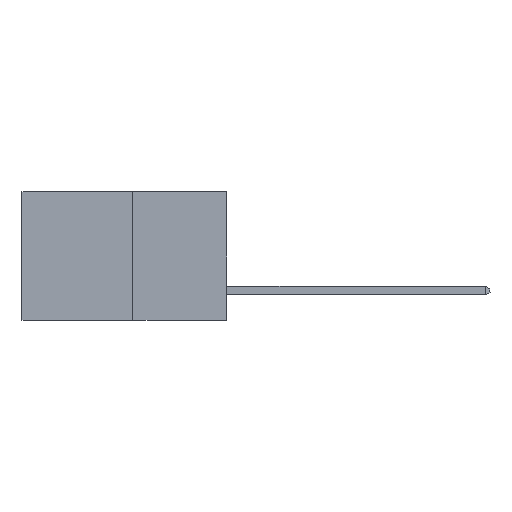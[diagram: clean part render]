
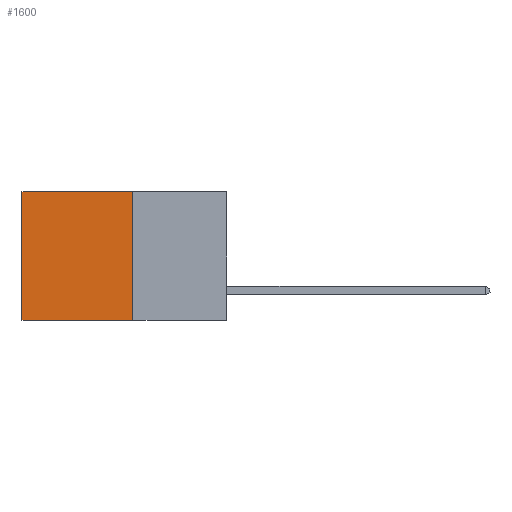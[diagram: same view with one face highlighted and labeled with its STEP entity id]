
A CAD part, left-side view. The second image highlights one B-rep face of the part: STEP entity #1600.
In plain terms, the highlighted planar face has unit normal (-1, 0, 0).
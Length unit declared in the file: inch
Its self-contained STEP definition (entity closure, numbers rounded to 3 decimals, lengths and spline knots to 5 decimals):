
#81 = EDGE_CURVE ( 'NONE', #3476, #1155, #4090, .T. ) ;
#1049 = ORIENTED_EDGE ( 'NONE', *, *, #2404, .T. ) ;
#1155 = VERTEX_POINT ( 'NONE', #3447 ) ;
#1250 = VECTOR ( 'NONE', #4417, 39.37008 ) ;
#1600 = ADVANCED_FACE ( 'NONE', ( #4902 ), #5461, .F. ) ;
#1651 = ORIENTED_EDGE ( 'NONE', *, *, #4720, .T. ) ;
#1663 = ORIENTED_EDGE ( 'NONE', *, *, #81, .F. ) ;
#1811 = VECTOR ( 'NONE', #3753, 39.37008 ) ;
#1872 = ORIENTED_EDGE ( 'NONE', *, *, #5780, .F. ) ;
#2404 = EDGE_CURVE ( 'NONE', #3476, #9478, #9103, .T. ) ;
#2645 = VECTOR ( 'NONE', #2736, 39.37008 ) ;
#2736 = DIRECTION ( 'NONE',  ( 0., 1., 0. ) ) ;
#3257 = VECTOR ( 'NONE', #9113, 39.37008 ) ;
#3447 = CARTESIAN_POINT ( 'NONE',  ( 0.277, 0.27, -0.37 ) ) ;
#3476 = VERTEX_POINT ( 'NONE', #9309 ) ;
#3636 = LINE ( 'NONE', #4492, #1250 ) ;
#3753 = DIRECTION ( 'NONE',  ( 0., 0., -1. ) ) ;
#4090 = LINE ( 'NONE', #5307, #1811 ) ;
#4417 = DIRECTION ( 'NONE',  ( 0., 0., -1. ) ) ;
#4492 = CARTESIAN_POINT ( 'NONE',  ( 0.277, 0.59, -0.37 ) ) ;
#4612 = CARTESIAN_POINT ( 'NONE',  ( 0.277, 0.27, -0.37 ) ) ;
#4720 = EDGE_CURVE ( 'NONE', #9478, #10011, #3636, .T. ) ;
#4902 = FACE_OUTER_BOUND ( 'NONE', #6759, .T. ) ;
#5194 = DIRECTION ( 'NONE',  ( 1., 0., 0. ) ) ;
#5307 = CARTESIAN_POINT ( 'NONE',  ( 0.277, 0.27, -0.37 ) ) ;
#5311 = CARTESIAN_POINT ( 'NONE',  ( 0.277, 0.27, -0.37 ) ) ;
#5461 = PLANE ( 'NONE',  #5673 ) ;
#5591 = LINE ( 'NONE', #5311, #3257 ) ;
#5673 = AXIS2_PLACEMENT_3D ( 'NONE', #4612, #5194, #8203 ) ;
#5780 = EDGE_CURVE ( 'NONE', #1155, #10011, #5591, .T. ) ;
#6759 = EDGE_LOOP ( 'NONE', ( #1651, #1872, #1663, #1049 ) ) ;
#7189 = CARTESIAN_POINT ( 'NONE',  ( 0.277, 0.59, 0. ) ) ;
#8203 = DIRECTION ( 'NONE',  ( 0., 0., -1. ) ) ;
#9098 = CARTESIAN_POINT ( 'NONE',  ( 0.277, 0.59, -0.37 ) ) ;
#9103 = LINE ( 'NONE', #9741, #2645 ) ;
#9113 = DIRECTION ( 'NONE',  ( 0., 1., 0. ) ) ;
#9309 = CARTESIAN_POINT ( 'NONE',  ( 0.277, 0.27, 0. ) ) ;
#9478 = VERTEX_POINT ( 'NONE', #7189 ) ;
#9741 = CARTESIAN_POINT ( 'NONE',  ( 0.277, 0.27, 0. ) ) ;
#10011 = VERTEX_POINT ( 'NONE', #9098 ) ;
